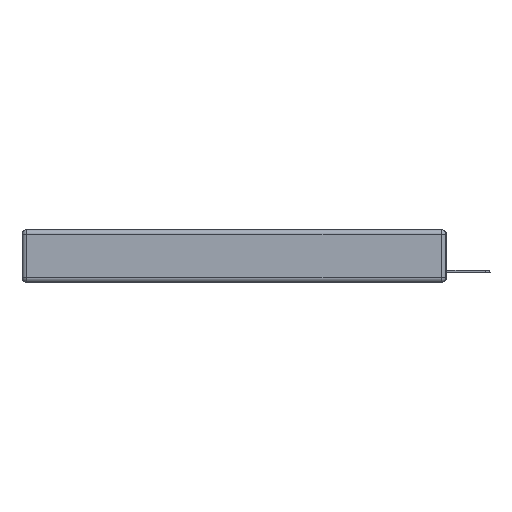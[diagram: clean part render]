
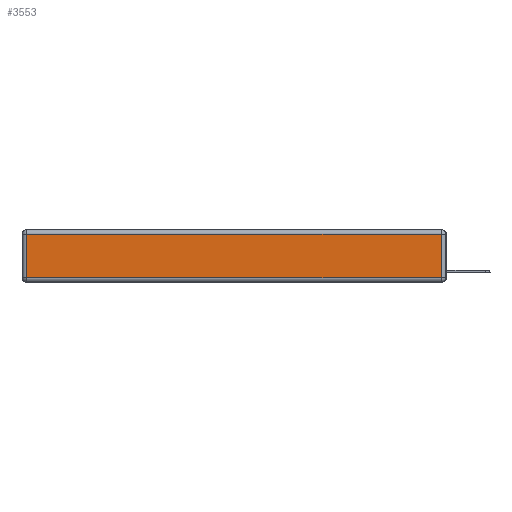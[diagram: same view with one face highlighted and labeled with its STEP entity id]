
A CAD part, left-side view. The second image highlights one B-rep face of the part: STEP entity #3553.
In plain terms, the highlighted planar face has unit normal (-1, 0, 0).
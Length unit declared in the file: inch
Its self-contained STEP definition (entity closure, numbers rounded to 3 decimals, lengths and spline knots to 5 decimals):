
#141 = EDGE_CURVE ( 'NONE', #3815, #1691, #16448, .T. ) ;
#875 = AXIS2_PLACEMENT_3D ( 'NONE', #17922, #1843, #11953 ) ;
#892 = CARTESIAN_POINT ( 'NONE',  ( 0., 2.72, -0.03 ) ) ;
#940 = VECTOR ( 'NONE', #15181, 39.37008 ) ;
#1691 = VERTEX_POINT ( 'NONE', #14528 ) ;
#1843 = DIRECTION ( 'NONE',  ( -1., 0., 0. ) ) ;
#1899 = VERTEX_POINT ( 'NONE', #13371 ) ;
#3553 = ADVANCED_FACE ( 'NONE', ( #16229 ), #10438, .T. ) ;
#3815 = VERTEX_POINT ( 'NONE', #892 ) ;
#4375 = VECTOR ( 'NONE', #5449, 39.37008 ) ;
#4399 = CARTESIAN_POINT ( 'NONE',  ( 0., 0.03, -0.03 ) ) ;
#4831 = LINE ( 'NONE', #9774, #4375 ) ;
#5449 = DIRECTION ( 'NONE',  ( 0., -1., 0. ) ) ;
#6259 = EDGE_CURVE ( 'NONE', #1899, #10612, #18448, .T. ) ;
#6310 = CARTESIAN_POINT ( 'NONE',  ( 0., 0.03, -0.343 ) ) ;
#6755 = ORIENTED_EDGE ( 'NONE', *, *, #8213, .T. ) ;
#8213 = EDGE_CURVE ( 'NONE', #10612, #3815, #9192, .T. ) ;
#8480 = EDGE_LOOP ( 'NONE', ( #17977, #10049, #6755, #12399 ) ) ;
#9192 = LINE ( 'NONE', #11670, #17222 ) ;
#9774 = CARTESIAN_POINT ( 'NONE',  ( 0., 0., -0.313 ) ) ;
#10049 = ORIENTED_EDGE ( 'NONE', *, *, #6259, .T. ) ;
#10438 = PLANE ( 'NONE',  #875 ) ;
#10612 = VERTEX_POINT ( 'NONE', #4399 ) ;
#11670 = CARTESIAN_POINT ( 'NONE',  ( 0., 2.75, -0.03 ) ) ;
#11953 = DIRECTION ( 'NONE',  ( 0., 0., 1. ) ) ;
#12399 = ORIENTED_EDGE ( 'NONE', *, *, #141, .T. ) ;
#13371 = CARTESIAN_POINT ( 'NONE',  ( 0., 0.03, -0.313 ) ) ;
#13753 = CARTESIAN_POINT ( 'NONE',  ( 0., 2.72, -0.343 ) ) ;
#14528 = CARTESIAN_POINT ( 'NONE',  ( 0., 2.72, -0.313 ) ) ;
#15181 = DIRECTION ( 'NONE',  ( 0., 0., -1. ) ) ;
#16083 = DIRECTION ( 'NONE',  ( 0., 1., 0. ) ) ;
#16229 = FACE_OUTER_BOUND ( 'NONE', #8480, .T. ) ;
#16448 = LINE ( 'NONE', #13753, #940 ) ;
#16545 = DIRECTION ( 'NONE',  ( 0., 0., 1. ) ) ;
#17222 = VECTOR ( 'NONE', #16083, 39.37008 ) ;
#17922 = CARTESIAN_POINT ( 'NONE',  ( 0., 0., -0.343 ) ) ;
#17976 = VECTOR ( 'NONE', #16545, 39.37008 ) ;
#17977 = ORIENTED_EDGE ( 'NONE', *, *, #18511, .T. ) ;
#18448 = LINE ( 'NONE', #6310, #17976 ) ;
#18511 = EDGE_CURVE ( 'NONE', #1691, #1899, #4831, .T. ) ;
